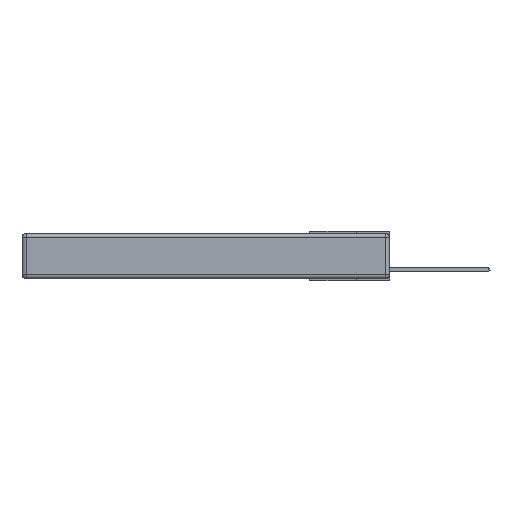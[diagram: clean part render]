
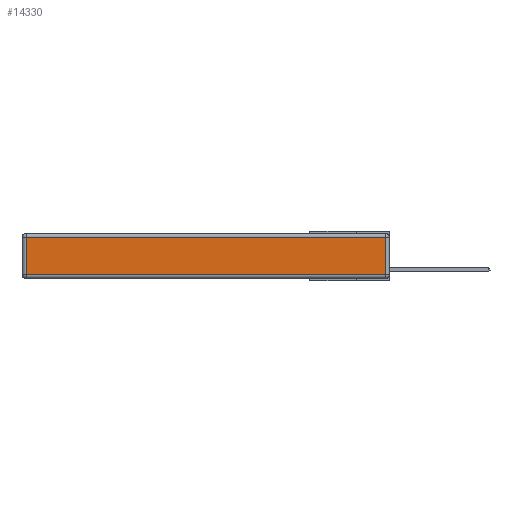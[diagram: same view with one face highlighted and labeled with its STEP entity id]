
A CAD part, left-side view. The second image highlights one B-rep face of the part: STEP entity #14330.
In plain terms, the highlighted planar face has unit normal (-1, 0, 0).
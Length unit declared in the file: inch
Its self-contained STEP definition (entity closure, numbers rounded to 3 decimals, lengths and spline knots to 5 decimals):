
#1578 = LINE ( 'NONE', #9025, #24726 ) ;
#1766 = VERTEX_POINT ( 'NONE', #21745 ) ;
#3069 = PLANE ( 'NONE',  #26514 ) ;
#3692 = LINE ( 'NONE', #21716, #18958 ) ;
#3963 = ORIENTED_EDGE ( 'NONE', *, *, #16851, .T. ) ;
#4736 = VECTOR ( 'NONE', #5545, 39.37008 ) ;
#5545 = DIRECTION ( 'NONE',  ( 0., -1., 0. ) ) ;
#5664 = DIRECTION ( 'NONE',  ( -1., 0., 0. ) ) ;
#5847 = ORIENTED_EDGE ( 'NONE', *, *, #18382, .T. ) ;
#6030 = EDGE_CURVE ( 'NONE', #19379, #1766, #1578, .T. ) ;
#6749 = CARTESIAN_POINT ( 'NONE',  ( 0., 0.03, -0.343 ) ) ;
#6962 = DIRECTION ( 'NONE',  ( 0., 1., 0. ) ) ;
#7457 = FACE_OUTER_BOUND ( 'NONE', #23168, .T. ) ;
#9025 = CARTESIAN_POINT ( 'NONE',  ( 0., 2.75, -0.03 ) ) ;
#9805 = CARTESIAN_POINT ( 'NONE',  ( 0., 0.03, -0.03 ) ) ;
#10289 = DIRECTION ( 'NONE',  ( 0., 0., -1. ) ) ;
#10502 = VECTOR ( 'NONE', #24937, 39.37008 ) ;
#11628 = CARTESIAN_POINT ( 'NONE',  ( 0., 2.72, -0.313 ) ) ;
#12423 = EDGE_CURVE ( 'NONE', #13709, #14563, #26071, .T. ) ;
#13709 = VERTEX_POINT ( 'NONE', #11628 ) ;
#14330 = ADVANCED_FACE ( 'NONE', ( #7457 ), #3069, .T. ) ;
#14395 = CARTESIAN_POINT ( 'NONE',  ( 0., 0., -0.343 ) ) ;
#14563 = VERTEX_POINT ( 'NONE', #17346 ) ;
#16851 = EDGE_CURVE ( 'NONE', #1766, #13709, #3692, .T. ) ;
#17346 = CARTESIAN_POINT ( 'NONE',  ( 0., 0.03, -0.313 ) ) ;
#18382 = EDGE_CURVE ( 'NONE', #14563, #19379, #22588, .T. ) ;
#18775 = ORIENTED_EDGE ( 'NONE', *, *, #6030, .T. ) ;
#18958 = VECTOR ( 'NONE', #10289, 39.37008 ) ;
#19167 = DIRECTION ( 'NONE',  ( 0., 0., 1. ) ) ;
#19379 = VERTEX_POINT ( 'NONE', #9805 ) ;
#21716 = CARTESIAN_POINT ( 'NONE',  ( 0., 2.72, -0.343 ) ) ;
#21745 = CARTESIAN_POINT ( 'NONE',  ( 0., 2.72, -0.03 ) ) ;
#22588 = LINE ( 'NONE', #6749, #10502 ) ;
#23168 = EDGE_LOOP ( 'NONE', ( #26556, #5847, #18775, #3963 ) ) ;
#23722 = CARTESIAN_POINT ( 'NONE',  ( 0., 0., -0.313 ) ) ;
#24726 = VECTOR ( 'NONE', #6962, 39.37008 ) ;
#24937 = DIRECTION ( 'NONE',  ( 0., 0., 1. ) ) ;
#26071 = LINE ( 'NONE', #23722, #4736 ) ;
#26514 = AXIS2_PLACEMENT_3D ( 'NONE', #14395, #5664, #19167 ) ;
#26556 = ORIENTED_EDGE ( 'NONE', *, *, #12423, .T. ) ;
